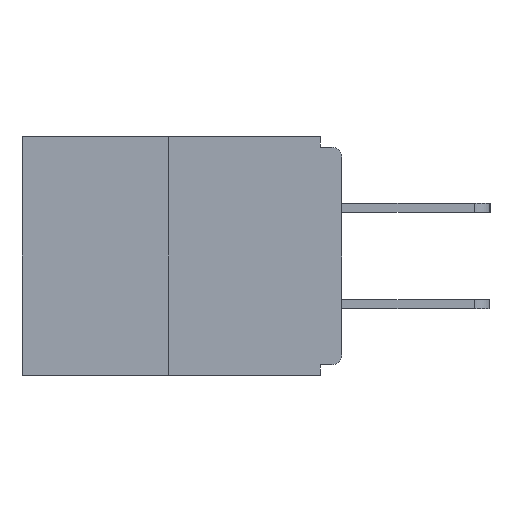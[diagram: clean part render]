
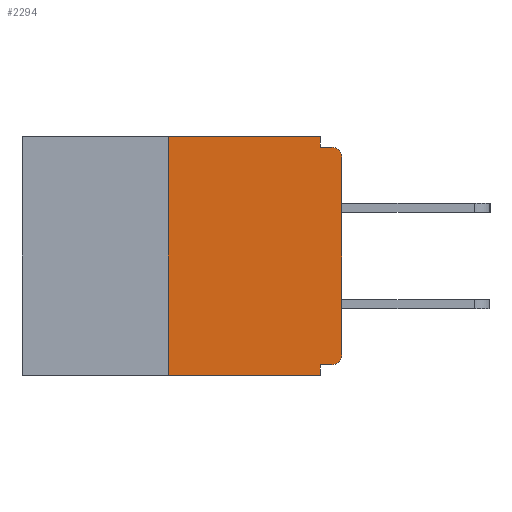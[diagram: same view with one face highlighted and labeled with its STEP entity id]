
A CAD part, left-side view. The second image highlights one B-rep face of the part: STEP entity #2294.
In plain terms, the highlighted planar face has unit normal (-1, 0, 0).
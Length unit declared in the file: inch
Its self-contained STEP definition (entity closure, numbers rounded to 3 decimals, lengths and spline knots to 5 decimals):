
#30 = LINE ( 'NONE', #8980, #14134 ) ;
#106 = VERTEX_POINT ( 'NONE', #9389 ) ;
#179 = CARTESIAN_POINT ( 'NONE',  ( 0., 0.031, -0.343 ) ) ;
#224 = DIRECTION ( 'NONE',  ( 0., -1., 0. ) ) ;
#456 = LINE ( 'NONE', #4064, #5076 ) ;
#464 = DIRECTION ( 'NONE',  ( -1., 0., 0. ) ) ;
#596 = CIRCLE ( 'NONE', #7656, 0.015 ) ;
#839 = DIRECTION ( 'NONE',  ( 0., 1., 0. ) ) ;
#1157 = EDGE_CURVE ( 'NONE', #14974, #7231, #15364, .T. ) ;
#1196 = LINE ( 'NONE', #9681, #2027 ) ;
#1378 = VERTEX_POINT ( 'NONE', #15556 ) ;
#1420 = DIRECTION ( 'NONE',  ( 0., 0., -1. ) ) ;
#1443 = CARTESIAN_POINT ( 'NONE',  ( 0., 0., -0.03 ) ) ;
#1480 = CARTESIAN_POINT ( 'NONE',  ( 0., 0.015, -0.03 ) ) ;
#1642 = AXIS2_PLACEMENT_3D ( 'NONE', #8761, #14303, #14182 ) ;
#1754 = EDGE_CURVE ( 'NONE', #17604, #1378, #596, .T. ) ;
#1776 = PLANE ( 'NONE',  #1642 ) ;
#2027 = VECTOR ( 'NONE', #224, 39.37008 ) ;
#2172 = EDGE_CURVE ( 'NONE', #3070, #1378, #1196, .T. ) ;
#2294 = ADVANCED_FACE ( 'NONE', ( #10608 ), #1776, .F. ) ;
#2664 = VECTOR ( 'NONE', #10843, 39.37008 ) ;
#2705 = CARTESIAN_POINT ( 'NONE',  ( 0., 0., 0. ) ) ;
#3070 = VERTEX_POINT ( 'NONE', #17573 ) ;
#3377 = EDGE_CURVE ( 'NONE', #106, #16732, #7787, .T. ) ;
#3638 = VECTOR ( 'NONE', #9308, 39.37008 ) ;
#4064 = CARTESIAN_POINT ( 'NONE',  ( 0., 0.25, 0. ) ) ;
#4652 = VECTOR ( 'NONE', #9887, 39.37008 ) ;
#5076 = VECTOR ( 'NONE', #17694, 39.37008 ) ;
#5342 = CARTESIAN_POINT ( 'NONE',  ( 0., 0.031, -0.343 ) ) ;
#5609 = DIRECTION ( 'NONE',  ( 0., 0., 1. ) ) ;
#5837 = VECTOR ( 'NONE', #5609, 39.37008 ) ;
#6017 = VERTEX_POINT ( 'NONE', #17358 ) ;
#6403 = ORIENTED_EDGE ( 'NONE', *, *, #15002, .F. ) ;
#6787 = DIRECTION ( 'NONE',  ( 0., 0., -1. ) ) ;
#7117 = ORIENTED_EDGE ( 'NONE', *, *, #1754, .T. ) ;
#7141 = EDGE_CURVE ( 'NONE', #16483, #8264, #11384, .T. ) ;
#7231 = VERTEX_POINT ( 'NONE', #9298 ) ;
#7656 = AXIS2_PLACEMENT_3D ( 'NONE', #1480, #15080, #6787 ) ;
#7787 = CIRCLE ( 'NONE', #11317, 0.015 ) ;
#8264 = VERTEX_POINT ( 'NONE', #179 ) ;
#8378 = VECTOR ( 'NONE', #1420, 39.37008 ) ;
#8560 = ORIENTED_EDGE ( 'NONE', *, *, #11544, .T. ) ;
#8561 = ORIENTED_EDGE ( 'NONE', *, *, #2172, .F. ) ;
#8761 = CARTESIAN_POINT ( 'NONE',  ( 0., 0.46, 0. ) ) ;
#8980 = CARTESIAN_POINT ( 'NONE',  ( 0., 0., -0.328 ) ) ;
#9136 = CARTESIAN_POINT ( 'NONE',  ( 0., 0., -0.313 ) ) ;
#9298 = CARTESIAN_POINT ( 'NONE',  ( 0., 0.031, 0. ) ) ;
#9308 = DIRECTION ( 'NONE',  ( 0., -1., 0. ) ) ;
#9389 = CARTESIAN_POINT ( 'NONE',  ( 0., 0.015, -0.328 ) ) ;
#9551 = CARTESIAN_POINT ( 'NONE',  ( 0., 0.46, -0.343 ) ) ;
#9681 = CARTESIAN_POINT ( 'NONE',  ( 0., 0., -0.015 ) ) ;
#9841 = ORIENTED_EDGE ( 'NONE', *, *, #17367, .F. ) ;
#9887 = DIRECTION ( 'NONE',  ( 0., 0., -1. ) ) ;
#10522 = EDGE_LOOP ( 'NONE', ( #13503, #6403, #11646, #11557, #9841, #13410, #8560, #7117, #8561, #12959 ) ) ;
#10608 = FACE_OUTER_BOUND ( 'NONE', #10522, .T. ) ;
#10843 = DIRECTION ( 'NONE',  ( 0., -1., 0. ) ) ;
#11317 = AXIS2_PLACEMENT_3D ( 'NONE', #14084, #464, #11530 ) ;
#11384 = LINE ( 'NONE', #9551, #3638 ) ;
#11530 = DIRECTION ( 'NONE',  ( 0., 0., -1. ) ) ;
#11544 = EDGE_CURVE ( 'NONE', #16732, #17604, #13196, .T. ) ;
#11557 = ORIENTED_EDGE ( 'NONE', *, *, #12615, .F. ) ;
#11646 = ORIENTED_EDGE ( 'NONE', *, *, #7141, .T. ) ;
#12177 = CARTESIAN_POINT ( 'NONE',  ( 0., 0.25, 0. ) ) ;
#12615 = EDGE_CURVE ( 'NONE', #6017, #8264, #15702, .T. ) ;
#12959 = ORIENTED_EDGE ( 'NONE', *, *, #15019, .F. ) ;
#13196 = LINE ( 'NONE', #2705, #5837 ) ;
#13410 = ORIENTED_EDGE ( 'NONE', *, *, #3377, .T. ) ;
#13503 = ORIENTED_EDGE ( 'NONE', *, *, #1157, .F. ) ;
#14084 = CARTESIAN_POINT ( 'NONE',  ( 0., 0.015, -0.313 ) ) ;
#14134 = VECTOR ( 'NONE', #839, 39.37008 ) ;
#14182 = DIRECTION ( 'NONE',  ( 0., 0., -1. ) ) ;
#14303 = DIRECTION ( 'NONE',  ( 1., 0., 0. ) ) ;
#14974 = VERTEX_POINT ( 'NONE', #12177 ) ;
#15002 = EDGE_CURVE ( 'NONE', #16483, #14974, #456, .T. ) ;
#15019 = EDGE_CURVE ( 'NONE', #7231, #3070, #16279, .T. ) ;
#15080 = DIRECTION ( 'NONE',  ( -1., 0., 0. ) ) ;
#15329 = CARTESIAN_POINT ( 'NONE',  ( 0., 0.25, -0.343 ) ) ;
#15364 = LINE ( 'NONE', #16282, #2664 ) ;
#15556 = CARTESIAN_POINT ( 'NONE',  ( 0., 0.015, -0.015 ) ) ;
#15702 = LINE ( 'NONE', #5342, #8378 ) ;
#16279 = LINE ( 'NONE', #16726, #4652 ) ;
#16282 = CARTESIAN_POINT ( 'NONE',  ( 0., 0.46, 0. ) ) ;
#16483 = VERTEX_POINT ( 'NONE', #15329 ) ;
#16726 = CARTESIAN_POINT ( 'NONE',  ( 0., 0.031, 0. ) ) ;
#16732 = VERTEX_POINT ( 'NONE', #9136 ) ;
#17358 = CARTESIAN_POINT ( 'NONE',  ( 0., 0.031, -0.328 ) ) ;
#17367 = EDGE_CURVE ( 'NONE', #106, #6017, #30, .T. ) ;
#17573 = CARTESIAN_POINT ( 'NONE',  ( 0., 0.031, -0.015 ) ) ;
#17604 = VERTEX_POINT ( 'NONE', #1443 ) ;
#17694 = DIRECTION ( 'NONE',  ( 0., 0., 1. ) ) ;
